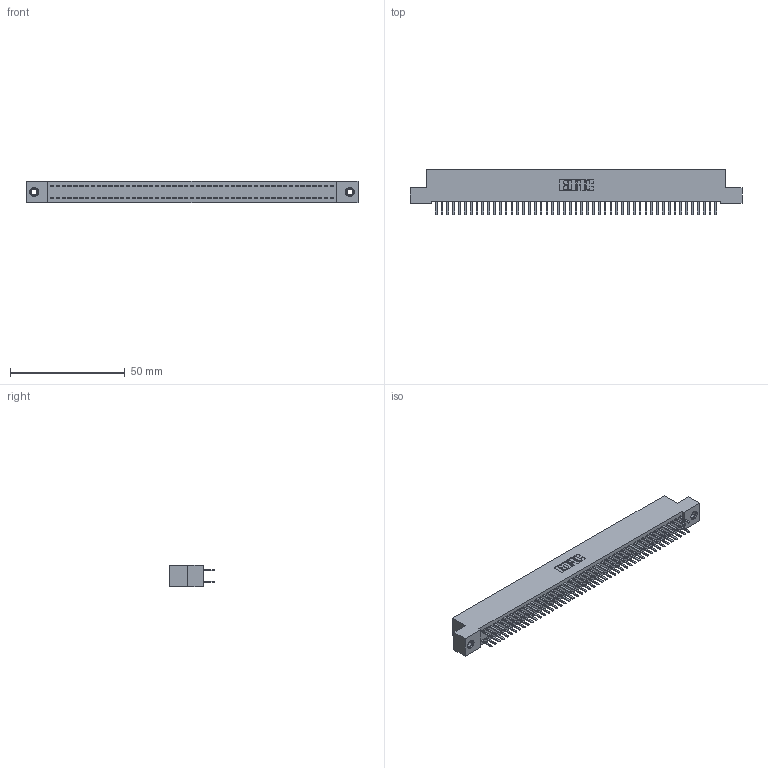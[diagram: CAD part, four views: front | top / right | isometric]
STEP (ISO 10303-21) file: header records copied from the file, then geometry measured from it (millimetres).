
FILE_DESCRIPTION (( 'STEP AP203' ), '1' );
FILE_NAME ('392-098-520-207.STEP', '2019-10-09T20:11:04', ( '' ), ( '' ), 'SwSTEP 2.0', 'SolidWorks 2016', '' );
FILE_SCHEMA (( 'CONFIG_CONTROL_DESIGN' ));
Length unit declared in the file: inch
Products named in the file (4): 392-098-520-207; 342 Part_TI; 345-292-001_345-293-120; 345-250-001_345-250-005-103
Assembly tree (101 placements, depth 2):
  392-098-520-207
    342 Part_TI
    345-292-001_345-293-120  x98
    345-250-001_345-250-005-103  x2
Bounding box: 144.78 x 20.02 x 9.4 mm (x, y, z)
Volume: 12985.8 mm3; surface area: 21234.3 mm2
Topology: 101 solids, 101 shells, 5658 faces, 16409 edges, 10670 vertices
Faces by surface type: plane 3822, cylinder 1820, cone 12, torus 4
Entity records: 31786 total; most frequent: CARTESIAN_POINT 5253, ORIENTED_EDGE 5170, DIRECTION 4495, EDGE_CURVE 2585, VECTOR 2433, LINE 2433, VERTEX_POINT 1716, AXIS2_PLACEMENT_3D 1031
